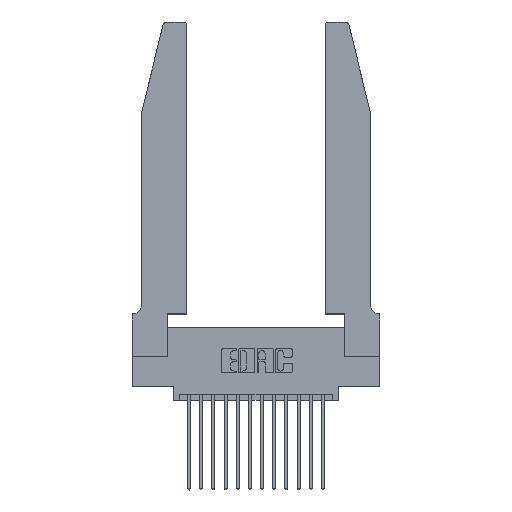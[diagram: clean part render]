
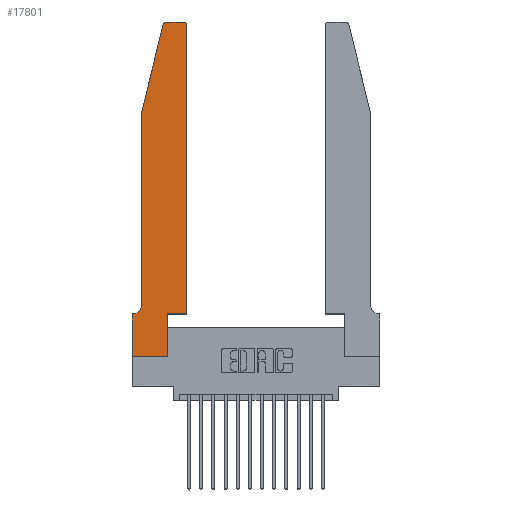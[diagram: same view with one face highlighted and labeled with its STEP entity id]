
A CAD part, top view. The second image highlights one B-rep face of the part: STEP entity #17801.
In plain terms, the highlighted planar face has unit normal (0, 0, 1).
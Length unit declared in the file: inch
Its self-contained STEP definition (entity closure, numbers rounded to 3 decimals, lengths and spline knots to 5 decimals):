
#155 = VECTOR ( 'NONE', #6908, 39.37008 ) ;
#445 = CARTESIAN_POINT ( 'NONE',  ( 0.284, 2.72, 0.37 ) ) ;
#477 = CARTESIAN_POINT ( 'NONE',  ( 0.4505, 0.35, 0.37 ) ) ;
#534 = VERTEX_POINT ( 'NONE', #2728 ) ;
#620 = DIRECTION ( 'NONE',  ( 0., 0., 1. ) ) ;
#627 = ORIENTED_EDGE ( 'NONE', *, *, #14090, .T. ) ;
#639 = LINE ( 'NONE', #16339, #9535 ) ;
#709 = PLANE ( 'NONE',  #15502 ) ;
#900 = DIRECTION ( 'NONE',  ( -1., 0., 0. ) ) ;
#1288 = VECTOR ( 'NONE', #3615, 39.37008 ) ;
#1812 = LINE ( 'NONE', #15979, #12919 ) ;
#1903 = EDGE_CURVE ( 'NONE', #14599, #5888, #3167, .T. ) ;
#2216 = DIRECTION ( 'NONE',  ( -1., 0., 0. ) ) ;
#2276 = CARTESIAN_POINT ( 'NONE',  ( 0.0055, 0.35, 0.37 ) ) ;
#2728 = CARTESIAN_POINT ( 'NONE',  ( 0.2865, 0., 0.37 ) ) ;
#2833 = LINE ( 'NONE', #13399, #1288 ) ;
#2856 = CARTESIAN_POINT ( 'NONE',  ( 0.4505, 0.35, 0.37 ) ) ;
#2885 = DIRECTION ( 'NONE',  ( -0.239, -0.971, 0. ) ) ;
#2982 = LINE ( 'NONE', #17637, #13835 ) ;
#3156 = CARTESIAN_POINT ( 'NONE',  ( 0.0755, 2., 0.37 ) ) ;
#3167 = CIRCLE ( 'NONE', #14716, 0.03 ) ;
#3168 = ORIENTED_EDGE ( 'NONE', *, *, #1903, .T. ) ;
#3292 = LINE ( 'NONE', #3156, #17927 ) ;
#3341 = VERTEX_POINT ( 'NONE', #17578 ) ;
#3402 = DIRECTION ( 'NONE',  ( 1., 0., 0. ) ) ;
#3586 = ORIENTED_EDGE ( 'NONE', *, *, #17038, .T. ) ;
#3615 = DIRECTION ( 'NONE',  ( -1., 0., 0. ) ) ;
#3652 = EDGE_LOOP ( 'NONE', ( #17167, #10550, #11282, #3586, #11624, #12471, #627, #4910, #8902, #6303, #13276, #3168 ) ) ;
#4910 = ORIENTED_EDGE ( 'NONE', *, *, #8699, .T. ) ;
#5162 = LINE ( 'NONE', #14626, #7181 ) ;
#5599 = VERTEX_POINT ( 'NONE', #14665 ) ;
#5772 = CARTESIAN_POINT ( 'NONE',  ( 0.0755, 0.42, 0.37 ) ) ;
#5888 = VERTEX_POINT ( 'NONE', #7836 ) ;
#6303 = ORIENTED_EDGE ( 'NONE', *, *, #13317, .T. ) ;
#6908 = DIRECTION ( 'NONE',  ( 0., 1., 0. ) ) ;
#7027 = DIRECTION ( 'NONE',  ( 1., 0., 0. ) ) ;
#7181 = VECTOR ( 'NONE', #13197, 39.37008 ) ;
#7249 = EDGE_CURVE ( 'NONE', #9961, #15041, #7695, .T. ) ;
#7260 = LINE ( 'NONE', #18056, #155 ) ;
#7435 = AXIS2_PLACEMENT_3D ( 'NONE', #445, #620, #7688 ) ;
#7688 = DIRECTION ( 'NONE',  ( 1., 0., 0. ) ) ;
#7695 = CIRCLE ( 'NONE', #7435, 0.03 ) ;
#7771 = EDGE_CURVE ( 'NONE', #12286, #12086, #17438, .T. ) ;
#7836 = CARTESIAN_POINT ( 'NONE',  ( 0.4205, 2.75, 0.37 ) ) ;
#8030 = AXIS2_PLACEMENT_3D ( 'NONE', #14809, #16369, #2216 ) ;
#8137 = CARTESIAN_POINT ( 'NONE',  ( 0., 0., 0.37 ) ) ;
#8143 = FACE_OUTER_BOUND ( 'NONE', #3652, .T. ) ;
#8517 = VECTOR ( 'NONE', #7027, 39.37008 ) ;
#8699 = EDGE_CURVE ( 'NONE', #9823, #534, #2982, .T. ) ;
#8902 = ORIENTED_EDGE ( 'NONE', *, *, #17956, .T. ) ;
#9399 = DIRECTION ( 'NONE',  ( 1., 0., 0. ) ) ;
#9444 = DIRECTION ( 'NONE',  ( 0., 0., 1. ) ) ;
#9511 = LINE ( 'NONE', #15851, #15716 ) ;
#9535 = VECTOR ( 'NONE', #900, 39.37008 ) ;
#9823 = VERTEX_POINT ( 'NONE', #8137 ) ;
#9961 = VERTEX_POINT ( 'NONE', #12723 ) ;
#10550 = ORIENTED_EDGE ( 'NONE', *, *, #7249, .T. ) ;
#10759 = CARTESIAN_POINT ( 'NONE',  ( 0.4205, 2.72, 0.37 ) ) ;
#11192 = EDGE_CURVE ( 'NONE', #15041, #5599, #9511, .T. ) ;
#11268 = CARTESIAN_POINT ( 'NONE',  ( 0.4505, 2.72, 0.37 ) ) ;
#11282 = ORIENTED_EDGE ( 'NONE', *, *, #11192, .T. ) ;
#11451 = EDGE_CURVE ( 'NONE', #5888, #9961, #2833, .T. ) ;
#11545 = DIRECTION ( 'NONE',  ( 0., -1., 0. ) ) ;
#11624 = ORIENTED_EDGE ( 'NONE', *, *, #7771, .T. ) ;
#12086 = VERTEX_POINT ( 'NONE', #2276 ) ;
#12286 = VERTEX_POINT ( 'NONE', #5772 ) ;
#12471 = ORIENTED_EDGE ( 'NONE', *, *, #16073, .T. ) ;
#12723 = CARTESIAN_POINT ( 'NONE',  ( 0.284, 2.75, 0.37 ) ) ;
#12919 = VECTOR ( 'NONE', #17144, 39.37008 ) ;
#13197 = DIRECTION ( 'NONE',  ( 0., 1., 0. ) ) ;
#13276 = ORIENTED_EDGE ( 'NONE', *, *, #13572, .T. ) ;
#13317 = EDGE_CURVE ( 'NONE', #3341, #17265, #15603, .T. ) ;
#13399 = CARTESIAN_POINT ( 'NONE',  ( 0.2605, 2.75, 0.37 ) ) ;
#13529 = DIRECTION ( 'NONE',  ( 0., 0., 1. ) ) ;
#13572 = EDGE_CURVE ( 'NONE', #17265, #14599, #5162, .T. ) ;
#13835 = VECTOR ( 'NONE', #3402, 39.37008 ) ;
#14090 = EDGE_CURVE ( 'NONE', #15978, #9823, #1812, .T. ) ;
#14599 = VERTEX_POINT ( 'NONE', #11268 ) ;
#14626 = CARTESIAN_POINT ( 'NONE',  ( 0.4505, 0.35, 0.37 ) ) ;
#14665 = CARTESIAN_POINT ( 'NONE',  ( 0.0755, 2., 0.37 ) ) ;
#14716 = AXIS2_PLACEMENT_3D ( 'NONE', #10759, #9444, #16321 ) ;
#14809 = CARTESIAN_POINT ( 'NONE',  ( 0.0055, 0.42, 0.37 ) ) ;
#15041 = VERTEX_POINT ( 'NONE', #15314 ) ;
#15314 = CARTESIAN_POINT ( 'NONE',  ( 0.25487, 2.72718, 0.37 ) ) ;
#15502 = AXIS2_PLACEMENT_3D ( 'NONE', #16514, #13529, #9399 ) ;
#15603 = LINE ( 'NONE', #2856, #8517 ) ;
#15716 = VECTOR ( 'NONE', #2885, 39.37008 ) ;
#15851 = CARTESIAN_POINT ( 'NONE',  ( 0.0755, 2., 0.37 ) ) ;
#15978 = VERTEX_POINT ( 'NONE', #16091 ) ;
#15979 = CARTESIAN_POINT ( 'NONE',  ( 0., 0., 0.37 ) ) ;
#16073 = EDGE_CURVE ( 'NONE', #12086, #15978, #639, .T. ) ;
#16091 = CARTESIAN_POINT ( 'NONE',  ( 0., 0.35, 0.37 ) ) ;
#16321 = DIRECTION ( 'NONE',  ( 1., 0., 0. ) ) ;
#16339 = CARTESIAN_POINT ( 'NONE',  ( 0.0755, 0.35, 0.37 ) ) ;
#16369 = DIRECTION ( 'NONE',  ( 0., 0., -1. ) ) ;
#16514 = CARTESIAN_POINT ( 'NONE',  ( 0., 0.35, 0.37 ) ) ;
#17038 = EDGE_CURVE ( 'NONE', #5599, #12286, #3292, .T. ) ;
#17144 = DIRECTION ( 'NONE',  ( 0., -1., 0. ) ) ;
#17167 = ORIENTED_EDGE ( 'NONE', *, *, #11451, .T. ) ;
#17265 = VERTEX_POINT ( 'NONE', #477 ) ;
#17438 = CIRCLE ( 'NONE', #8030, 0.07 ) ;
#17578 = CARTESIAN_POINT ( 'NONE',  ( 0.2865, 0.35, 0.37 ) ) ;
#17637 = CARTESIAN_POINT ( 'NONE',  ( 0., 0., 0.37 ) ) ;
#17801 = ADVANCED_FACE ( 'NONE', ( #8143 ), #709, .T. ) ;
#17927 = VECTOR ( 'NONE', #11545, 39.37008 ) ;
#17956 = EDGE_CURVE ( 'NONE', #534, #3341, #7260, .T. ) ;
#18056 = CARTESIAN_POINT ( 'NONE',  ( 0.2865, 0.35, 0.37 ) ) ;
